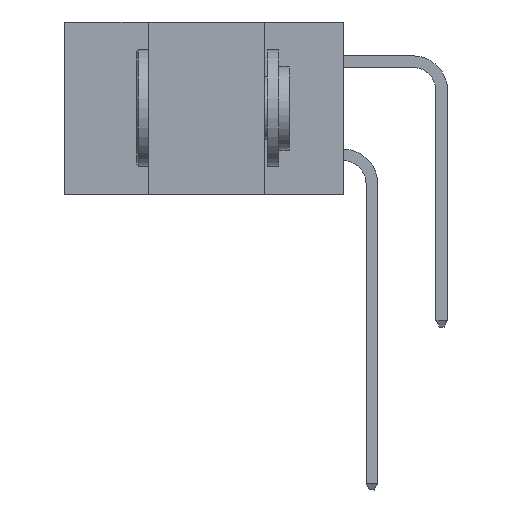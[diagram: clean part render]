
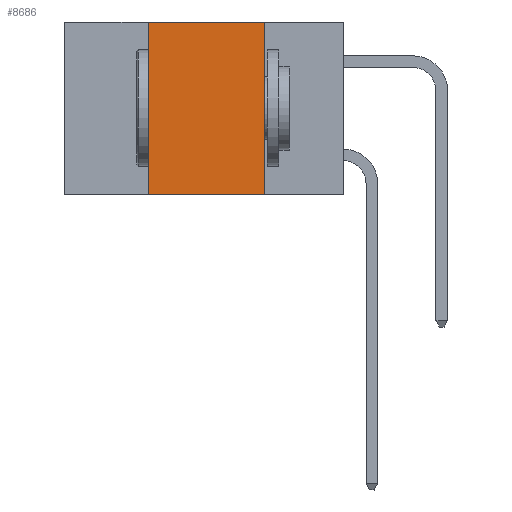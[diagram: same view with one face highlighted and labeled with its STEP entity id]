
A CAD part, left-side view. The second image highlights one B-rep face of the part: STEP entity #8686.
In plain terms, the highlighted planar face has unit normal (-1, 0, 0).
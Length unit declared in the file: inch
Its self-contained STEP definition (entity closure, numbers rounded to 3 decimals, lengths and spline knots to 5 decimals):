
#1348 = DIRECTION ( 'NONE',  ( 1., 0., 0. ) ) ;
#1746 = ORIENTED_EDGE ( 'NONE', *, *, #10956, .F. ) ;
#1891 = CARTESIAN_POINT ( 'NONE',  ( 0., 0.17, 0. ) ) ;
#1916 = LINE ( 'NONE', #5796, #12976 ) ;
#1993 = EDGE_CURVE ( 'NONE', #11429, #10100, #11243, .T. ) ;
#2229 = VERTEX_POINT ( 'NONE', #6969 ) ;
#2348 = PLANE ( 'NONE',  #8622 ) ;
#2362 = CARTESIAN_POINT ( 'NONE',  ( 0., 0.42, -0.37 ) ) ;
#2416 = ORIENTED_EDGE ( 'NONE', *, *, #1993, .F. ) ;
#3369 = CARTESIAN_POINT ( 'NONE',  ( 0., 0.42, 0. ) ) ;
#3544 = FACE_OUTER_BOUND ( 'NONE', #9082, .T. ) ;
#3812 = CARTESIAN_POINT ( 'NONE',  ( 0., 0.6, 0. ) ) ;
#4405 = VECTOR ( 'NONE', #12984, 39.37008 ) ;
#5166 = EDGE_CURVE ( 'NONE', #6914, #2229, #8909, .T. ) ;
#5796 = CARTESIAN_POINT ( 'NONE',  ( 0., 0.6, -0.37 ) ) ;
#6914 = VERTEX_POINT ( 'NONE', #1891 ) ;
#6969 = CARTESIAN_POINT ( 'NONE',  ( 0., 0.17, -0.37 ) ) ;
#7011 = CARTESIAN_POINT ( 'NONE',  ( 0., 0.42, -0.37 ) ) ;
#7453 = DIRECTION ( 'NONE',  ( 0., 0., 1. ) ) ;
#7627 = CARTESIAN_POINT ( 'NONE',  ( 0., 0.6, 0. ) ) ;
#8622 = AXIS2_PLACEMENT_3D ( 'NONE', #7627, #1348, #11686 ) ;
#8686 = ADVANCED_FACE ( 'NONE', ( #3544 ), #2348, .F. ) ;
#8909 = LINE ( 'NONE', #10911, #4405 ) ;
#8987 = DIRECTION ( 'NONE',  ( 0., -1., 0. ) ) ;
#9082 = EDGE_LOOP ( 'NONE', ( #11095, #1746, #2416, #12015 ) ) ;
#9885 = LINE ( 'NONE', #3812, #12935 ) ;
#10100 = VERTEX_POINT ( 'NONE', #3369 ) ;
#10911 = CARTESIAN_POINT ( 'NONE',  ( 0., 0.17, -0.37 ) ) ;
#10956 = EDGE_CURVE ( 'NONE', #10100, #6914, #9885, .T. ) ;
#11090 = DIRECTION ( 'NONE',  ( 0., -1., 0. ) ) ;
#11095 = ORIENTED_EDGE ( 'NONE', *, *, #5166, .F. ) ;
#11243 = LINE ( 'NONE', #2362, #13089 ) ;
#11429 = VERTEX_POINT ( 'NONE', #7011 ) ;
#11686 = DIRECTION ( 'NONE',  ( 0., 0., -1. ) ) ;
#12015 = ORIENTED_EDGE ( 'NONE', *, *, #13033, .T. ) ;
#12935 = VECTOR ( 'NONE', #11090, 39.37008 ) ;
#12976 = VECTOR ( 'NONE', #8987, 39.37008 ) ;
#12984 = DIRECTION ( 'NONE',  ( 0., 0., -1. ) ) ;
#13033 = EDGE_CURVE ( 'NONE', #11429, #2229, #1916, .T. ) ;
#13089 = VECTOR ( 'NONE', #7453, 39.37008 ) ;
